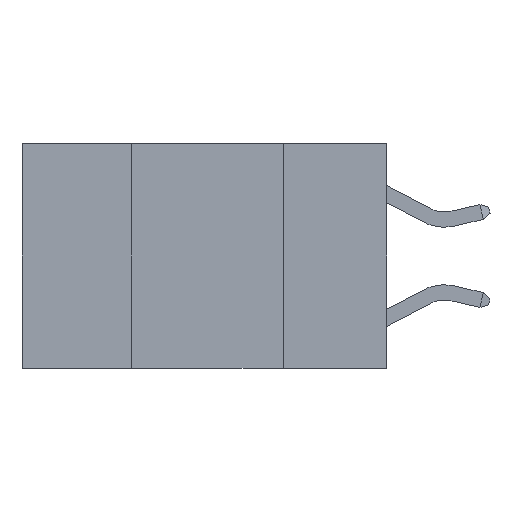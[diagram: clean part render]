
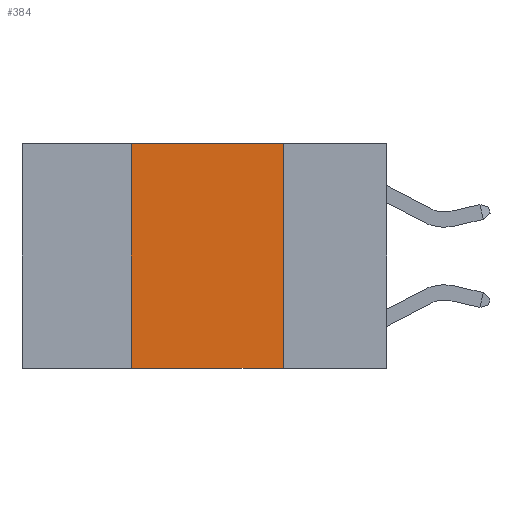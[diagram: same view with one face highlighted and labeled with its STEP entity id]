
A CAD part, left-side view. The second image highlights one B-rep face of the part: STEP entity #384.
In plain terms, the highlighted planar face has unit normal (-1, 0, 0).
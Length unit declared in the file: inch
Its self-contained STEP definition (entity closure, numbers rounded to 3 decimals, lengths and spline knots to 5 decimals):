
#252 = ORIENTED_EDGE ( 'NONE', *, *, #15676, .F. ) ;
#384 = ADVANCED_FACE ( 'NONE', ( #7291 ), #3728, .F. ) ;
#408 = CARTESIAN_POINT ( 'NONE',  ( 0., 0.17, 0. ) ) ;
#1148 = CARTESIAN_POINT ( 'NONE',  ( 0., 0.42, 0. ) ) ;
#1906 = DIRECTION ( 'NONE',  ( 0., 0., -1. ) ) ;
#2291 = CARTESIAN_POINT ( 'NONE',  ( 0., 0.6, 0. ) ) ;
#2411 = VERTEX_POINT ( 'NONE', #4075 ) ;
#2654 = VERTEX_POINT ( 'NONE', #4631 ) ;
#3256 = LINE ( 'NONE', #17701, #18062 ) ;
#3728 = PLANE ( 'NONE',  #7349 ) ;
#4075 = CARTESIAN_POINT ( 'NONE',  ( 0., 0.42, -0.37 ) ) ;
#4631 = CARTESIAN_POINT ( 'NONE',  ( 0., 0.17, 0. ) ) ;
#5186 = DIRECTION ( 'NONE',  ( 0., 0., -1. ) ) ;
#5834 = LINE ( 'NONE', #12722, #16837 ) ;
#7291 = FACE_OUTER_BOUND ( 'NONE', #14125, .T. ) ;
#7349 = AXIS2_PLACEMENT_3D ( 'NONE', #2291, #9492, #5186 ) ;
#8003 = ORIENTED_EDGE ( 'NONE', *, *, #11200, .F. ) ;
#8453 = ORIENTED_EDGE ( 'NONE', *, *, #17492, .T. ) ;
#9181 = DIRECTION ( 'NONE',  ( 0., -1., 0. ) ) ;
#9492 = DIRECTION ( 'NONE',  ( 1., 0., 0. ) ) ;
#10241 = VECTOR ( 'NONE', #14310, 39.37008 ) ;
#11047 = VECTOR ( 'NONE', #1906, 39.37008 ) ;
#11122 = VERTEX_POINT ( 'NONE', #1148 ) ;
#11200 = EDGE_CURVE ( 'NONE', #2411, #11122, #14039, .T. ) ;
#11925 = CARTESIAN_POINT ( 'NONE',  ( 0., 0.17, -0.37 ) ) ;
#12722 = CARTESIAN_POINT ( 'NONE',  ( 0., 0.6, -0.37 ) ) ;
#12884 = CARTESIAN_POINT ( 'NONE',  ( 0., 0.42, 0. ) ) ;
#13812 = EDGE_CURVE ( 'NONE', #2654, #14435, #18562, .T. ) ;
#14039 = LINE ( 'NONE', #12884, #10241 ) ;
#14125 = EDGE_LOOP ( 'NONE', ( #15164, #252, #8003, #8453 ) ) ;
#14154 = DIRECTION ( 'NONE',  ( 0., -1., 0. ) ) ;
#14310 = DIRECTION ( 'NONE',  ( 0., 0., 1. ) ) ;
#14435 = VERTEX_POINT ( 'NONE', #11925 ) ;
#15164 = ORIENTED_EDGE ( 'NONE', *, *, #13812, .F. ) ;
#15676 = EDGE_CURVE ( 'NONE', #11122, #2654, #3256, .T. ) ;
#16837 = VECTOR ( 'NONE', #14154, 39.37008 ) ;
#17492 = EDGE_CURVE ( 'NONE', #2411, #14435, #5834, .T. ) ;
#17701 = CARTESIAN_POINT ( 'NONE',  ( 0., 0.6, 0. ) ) ;
#18062 = VECTOR ( 'NONE', #9181, 39.37008 ) ;
#18562 = LINE ( 'NONE', #408, #11047 ) ;
